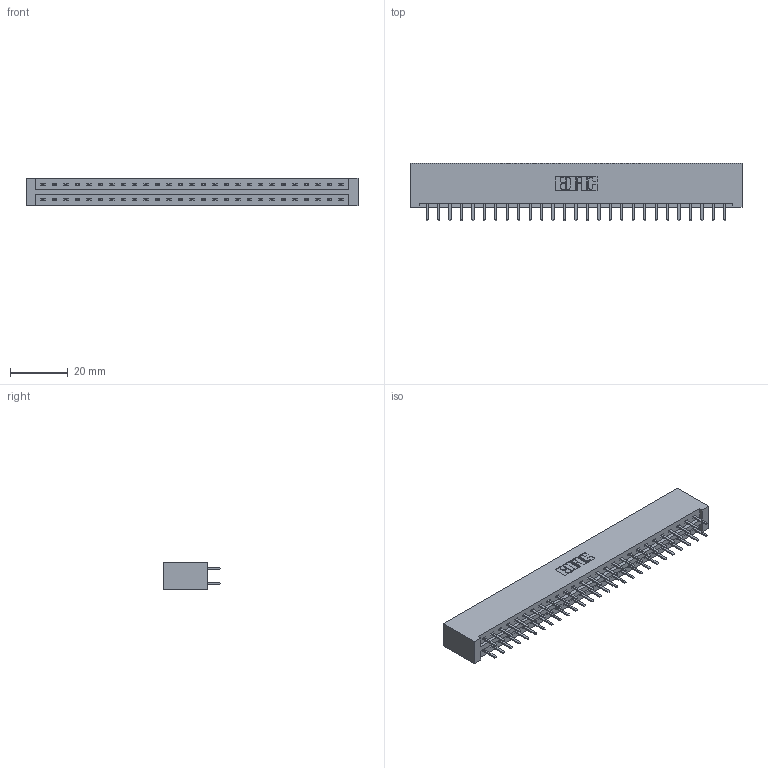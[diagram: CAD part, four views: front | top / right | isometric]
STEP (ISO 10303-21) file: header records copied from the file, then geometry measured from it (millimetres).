
FILE_DESCRIPTION (( 'STEP AP203' ), '1' );
FILE_NAME ('337-054-520-201.STEP', '2018-08-10T00:04:53', ( '' ), ( '' ), 'SwSTEP 2.0', 'SolidWorks 2016', '' );
FILE_SCHEMA (( 'CONFIG_CONTROL_DESIGN' ));
Length unit declared in the file: inch
Products named in the file (3): 337 Part_No Mounting Lugs; 345-292-001_345-293-120; 337-054-520-201
Assembly tree (55 placements, depth 2):
  337-054-520-201
    337 Part_No Mounting Lugs
    345-292-001_345-293-120  x54
Bounding box: 114.86 x 20.02 x 9.4 mm (x, y, z)
Volume: 12642.1 mm3; surface area: 14134.6 mm2
Topology: 55 solids, 55 shells, 3238 faces, 9413 edges, 6130 vertices
Faces by surface type: plane 2226, cylinder 1012
Entity records: 22711 total; most frequent: CARTESIAN_POINT 3850, ORIENTED_EDGE 3774, DIRECTION 3283, EDGE_CURVE 1887, VECTOR 1763, LINE 1763, VERTEX_POINT 1254, AXIS2_PLACEMENT_3D 760
